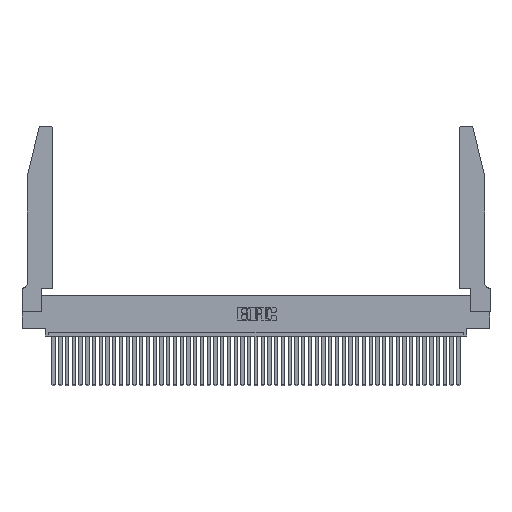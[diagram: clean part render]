
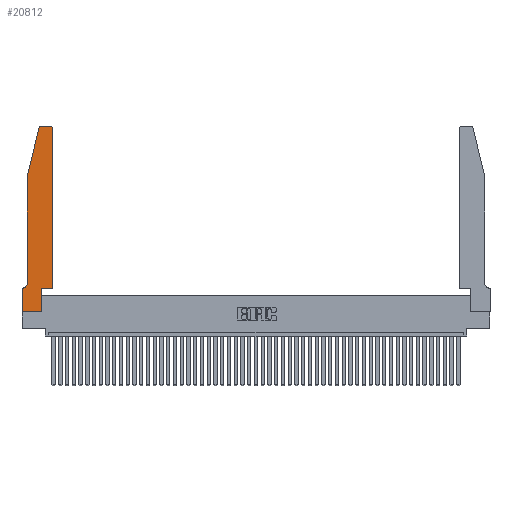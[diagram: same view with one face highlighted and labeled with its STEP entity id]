
A CAD part, top view. The second image highlights one B-rep face of the part: STEP entity #20812.
In plain terms, the highlighted planar face has unit normal (0, 0, 1).
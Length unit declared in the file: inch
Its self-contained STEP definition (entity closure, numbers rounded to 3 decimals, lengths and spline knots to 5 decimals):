
#399 = VECTOR ( 'NONE', #44882, 39.37008 ) ;
#606 = VECTOR ( 'NONE', #42439, 39.37008 ) ;
#1288 = DIRECTION ( 'NONE',  ( 0., 0., 1. ) ) ;
#1996 = CARTESIAN_POINT ( 'NONE',  ( 0.0055, 0.35, 0.37 ) ) ;
#2199 = CARTESIAN_POINT ( 'NONE',  ( 0., 0.35, 0.37 ) ) ;
#2405 = DIRECTION ( 'NONE',  ( 0., -1., 0. ) ) ;
#2637 = VERTEX_POINT ( 'NONE', #37952 ) ;
#3200 = VECTOR ( 'NONE', #2405, 39.37008 ) ;
#3306 = DIRECTION ( 'NONE',  ( 0., 1., 0. ) ) ;
#4249 = CARTESIAN_POINT ( 'NONE',  ( 0.4205, 2.75, 0.37 ) ) ;
#4789 = AXIS2_PLACEMENT_3D ( 'NONE', #38638, #27536, #12947 ) ;
#5050 = LINE ( 'NONE', #37953, #24189 ) ;
#5321 = CARTESIAN_POINT ( 'NONE',  ( 0.4205, 2.72, 0.37 ) ) ;
#5513 = VERTEX_POINT ( 'NONE', #27421 ) ;
#5865 = EDGE_CURVE ( 'NONE', #5513, #12104, #32413, .T. ) ;
#6269 = VECTOR ( 'NONE', #3306, 39.37008 ) ;
#7396 = VERTEX_POINT ( 'NONE', #20208 ) ;
#7444 = EDGE_CURVE ( 'NONE', #41706, #42323, #5050, .T. ) ;
#8602 = EDGE_CURVE ( 'NONE', #11514, #41706, #40959, .T. ) ;
#9062 = DIRECTION ( 'NONE',  ( 1., 0., 0. ) ) ;
#9962 = ORIENTED_EDGE ( 'NONE', *, *, #44064, .T. ) ;
#11514 = VERTEX_POINT ( 'NONE', #2199 ) ;
#11871 = ORIENTED_EDGE ( 'NONE', *, *, #7444, .T. ) ;
#11986 = ORIENTED_EDGE ( 'NONE', *, *, #16244, .T. ) ;
#12104 = VERTEX_POINT ( 'NONE', #23235 ) ;
#12287 = CARTESIAN_POINT ( 'NONE',  ( 0., 0.35, 0.37 ) ) ;
#12361 = EDGE_CURVE ( 'NONE', #40981, #34499, #26131, .T. ) ;
#12895 = ORIENTED_EDGE ( 'NONE', *, *, #37893, .T. ) ;
#12947 = DIRECTION ( 'NONE',  ( -1., 0., 0. ) ) ;
#13569 = VECTOR ( 'NONE', #40768, 39.37008 ) ;
#13708 = ORIENTED_EDGE ( 'NONE', *, *, #28449, .T. ) ;
#14435 = LINE ( 'NONE', #46989, #42332 ) ;
#15494 = CARTESIAN_POINT ( 'NONE',  ( 0.0755, 2., 0.37 ) ) ;
#15864 = EDGE_CURVE ( 'NONE', #28442, #40981, #33872, .T. ) ;
#16009 = DIRECTION ( 'NONE',  ( 1., 0., 0. ) ) ;
#16244 = EDGE_CURVE ( 'NONE', #7396, #5513, #21617, .T. ) ;
#16298 = LINE ( 'NONE', #37541, #606 ) ;
#17610 = CARTESIAN_POINT ( 'NONE',  ( 0.2605, 2.75, 0.37 ) ) ;
#17674 = EDGE_CURVE ( 'NONE', #12104, #28442, #24508, .T. ) ;
#17939 = DIRECTION ( 'NONE',  ( -1., 0., 0. ) ) ;
#18212 = AXIS2_PLACEMENT_3D ( 'NONE', #19926, #1288, #31001 ) ;
#18739 = AXIS2_PLACEMENT_3D ( 'NONE', #12287, #38321, #16009 ) ;
#19926 = CARTESIAN_POINT ( 'NONE',  ( 0.284, 2.72, 0.37 ) ) ;
#20208 = CARTESIAN_POINT ( 'NONE',  ( 0.2865, 0.35, 0.37 ) ) ;
#20715 = EDGE_CURVE ( 'NONE', #35594, #2637, #24019, .T. ) ;
#20812 = ADVANCED_FACE ( 'NONE', ( #25728 ), #34541, .T. ) ;
#21617 = LINE ( 'NONE', #40313, #13569 ) ;
#23235 = CARTESIAN_POINT ( 'NONE',  ( 0.4505, 2.72, 0.37 ) ) ;
#24019 = LINE ( 'NONE', #24224, #29788 ) ;
#24189 = VECTOR ( 'NONE', #33847, 39.37008 ) ;
#24224 = CARTESIAN_POINT ( 'NONE',  ( 0.0755, 2., 0.37 ) ) ;
#24242 = ORIENTED_EDGE ( 'NONE', *, *, #36714, .T. ) ;
#24479 = CARTESIAN_POINT ( 'NONE',  ( 0., 0., 0.37 ) ) ;
#24508 = CIRCLE ( 'NONE', #32364, 0.03 ) ;
#25048 = ORIENTED_EDGE ( 'NONE', *, *, #17674, .T. ) ;
#25728 = FACE_OUTER_BOUND ( 'NONE', #26324, .T. ) ;
#26131 = CIRCLE ( 'NONE', #18212, 0.03 ) ;
#26324 = EDGE_LOOP ( 'NONE', ( #31521, #43814, #12895, #46784, #24242, #13708, #47805, #11871, #9962, #11986, #26549, #25048 ) ) ;
#26549 = ORIENTED_EDGE ( 'NONE', *, *, #5865, .T. ) ;
#27421 = CARTESIAN_POINT ( 'NONE',  ( 0.4505, 0.35, 0.37 ) ) ;
#27536 = DIRECTION ( 'NONE',  ( 0., 0., -1. ) ) ;
#28442 = VERTEX_POINT ( 'NONE', #4249 ) ;
#28449 = EDGE_CURVE ( 'NONE', #46785, #11514, #16298, .T. ) ;
#29462 = CARTESIAN_POINT ( 'NONE',  ( 0.0755, 2., 0.37 ) ) ;
#29788 = VECTOR ( 'NONE', #32320, 39.37008 ) ;
#30363 = CARTESIAN_POINT ( 'NONE',  ( 0.2865, 0., 0.37 ) ) ;
#31001 = DIRECTION ( 'NONE',  ( 1., 0., 0. ) ) ;
#31274 = DIRECTION ( 'NONE',  ( 0., 0., 1. ) ) ;
#31521 = ORIENTED_EDGE ( 'NONE', *, *, #15864, .T. ) ;
#32320 = DIRECTION ( 'NONE',  ( 0., -1., 0. ) ) ;
#32364 = AXIS2_PLACEMENT_3D ( 'NONE', #5321, #31274, #9062 ) ;
#32413 = LINE ( 'NONE', #36295, #6269 ) ;
#33237 = CARTESIAN_POINT ( 'NONE',  ( 0., 0., 0.37 ) ) ;
#33847 = DIRECTION ( 'NONE',  ( 1., 0., 0. ) ) ;
#33872 = LINE ( 'NONE', #17610, #46713 ) ;
#34499 = VERTEX_POINT ( 'NONE', #42511 ) ;
#34541 = PLANE ( 'NONE',  #18739 ) ;
#35074 = CIRCLE ( 'NONE', #4789, 0.07 ) ;
#35594 = VERTEX_POINT ( 'NONE', #15494 ) ;
#36295 = CARTESIAN_POINT ( 'NONE',  ( 0.4505, 0.35, 0.37 ) ) ;
#36714 = EDGE_CURVE ( 'NONE', #2637, #46785, #35074, .T. ) ;
#36997 = LINE ( 'NONE', #29462, #399 ) ;
#37541 = CARTESIAN_POINT ( 'NONE',  ( 0.0755, 0.35, 0.37 ) ) ;
#37893 = EDGE_CURVE ( 'NONE', #34499, #35594, #36997, .T. ) ;
#37952 = CARTESIAN_POINT ( 'NONE',  ( 0.0755, 0.42, 0.37 ) ) ;
#37953 = CARTESIAN_POINT ( 'NONE',  ( 0., 0., 0.37 ) ) ;
#38321 = DIRECTION ( 'NONE',  ( 0., 0., 1. ) ) ;
#38638 = CARTESIAN_POINT ( 'NONE',  ( 0.0055, 0.42, 0.37 ) ) ;
#39375 = DIRECTION ( 'NONE',  ( 0., 1., 0. ) ) ;
#40313 = CARTESIAN_POINT ( 'NONE',  ( 0.4505, 0.35, 0.37 ) ) ;
#40768 = DIRECTION ( 'NONE',  ( 1., 0., 0. ) ) ;
#40959 = LINE ( 'NONE', #24479, #3200 ) ;
#40981 = VERTEX_POINT ( 'NONE', #43617 ) ;
#41706 = VERTEX_POINT ( 'NONE', #33237 ) ;
#42323 = VERTEX_POINT ( 'NONE', #30363 ) ;
#42332 = VECTOR ( 'NONE', #39375, 39.37008 ) ;
#42439 = DIRECTION ( 'NONE',  ( -1., 0., 0. ) ) ;
#42511 = CARTESIAN_POINT ( 'NONE',  ( 0.25487, 2.72718, 0.37 ) ) ;
#43617 = CARTESIAN_POINT ( 'NONE',  ( 0.284, 2.75, 0.37 ) ) ;
#43814 = ORIENTED_EDGE ( 'NONE', *, *, #12361, .T. ) ;
#44064 = EDGE_CURVE ( 'NONE', #42323, #7396, #14435, .T. ) ;
#44882 = DIRECTION ( 'NONE',  ( -0.239, -0.971, 0. ) ) ;
#46713 = VECTOR ( 'NONE', #17939, 39.37008 ) ;
#46784 = ORIENTED_EDGE ( 'NONE', *, *, #20715, .T. ) ;
#46785 = VERTEX_POINT ( 'NONE', #1996 ) ;
#46989 = CARTESIAN_POINT ( 'NONE',  ( 0.2865, 0.35, 0.37 ) ) ;
#47805 = ORIENTED_EDGE ( 'NONE', *, *, #8602, .T. ) ;
